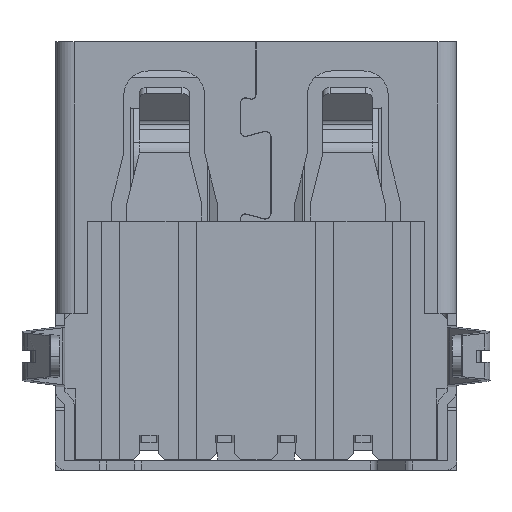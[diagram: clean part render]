
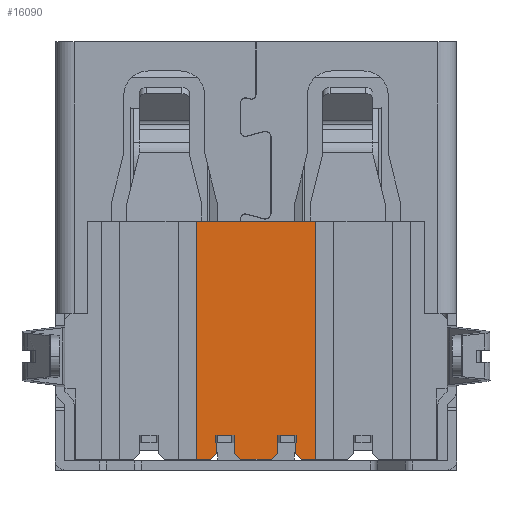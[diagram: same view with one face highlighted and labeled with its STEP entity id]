
A CAD part, front view. The second image highlights one B-rep face of the part: STEP entity #16090.
In plain terms, the highlighted planar face has unit normal (0, -1, 0).
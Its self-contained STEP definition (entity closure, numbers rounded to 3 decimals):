
#29 = DIRECTION ( 'NONE',  ( 1., 0., 0. ) ) ;
#78 = LINE ( 'NONE', #5264, #2960 ) ;
#275 = EDGE_CURVE ( 'NONE', #8951, #6910, #13512, .T. ) ;
#581 = CARTESIAN_POINT ( 'NONE',  ( 3.98, -6.1, 6.95 ) ) ;
#896 = CARTESIAN_POINT ( 'NONE',  ( -3.02, -6.1, 4.3 ) ) ;
#1021 = VERTEX_POINT ( 'NONE', #1642 ) ;
#1056 = VERTEX_POINT ( 'NONE', #20363 ) ;
#1101 = VECTOR ( 'NONE', #15560, 1000. ) ;
#1265 = LINE ( 'NONE', #12052, #1101 ) ;
#1316 = CARTESIAN_POINT ( 'NONE',  ( 4.77, -6.1, 7.75 ) ) ;
#1438 = CARTESIAN_POINT ( 'NONE',  ( 3.98, -6.1, 0. ) ) ;
#1642 = CARTESIAN_POINT ( 'NONE',  ( 4.57, -6.1, 5.55 ) ) ;
#1750 = CARTESIAN_POINT ( 'NONE',  ( 4.77, -6.1, 4.75 ) ) ;
#1772 = CARTESIAN_POINT ( 'NONE',  ( 4.77, -6.1, 4.75 ) ) ;
#1869 = DIRECTION ( 'NONE',  ( 0., 0., -1. ) ) ;
#2096 = ORIENTED_EDGE ( 'NONE', *, *, #8460, .T. ) ;
#2363 = ORIENTED_EDGE ( 'NONE', *, *, #4243, .T. ) ;
#2655 = DIRECTION ( 'NONE',  ( 0., 0., -1. ) ) ;
#2670 = VECTOR ( 'NONE', #2655, 1000. ) ;
#2960 = VECTOR ( 'NONE', #1869, 1000. ) ;
#3129 = VECTOR ( 'NONE', #16222, 1000. ) ;
#3176 = VECTOR ( 'NONE', #18240, 1000. ) ;
#3221 = CARTESIAN_POINT ( 'NONE',  ( 4.57, -6.1, 6.95 ) ) ;
#3343 = EDGE_CURVE ( 'NONE', #1056, #14543, #18358, .T. ) ;
#3367 = LINE ( 'NONE', #1438, #10193 ) ;
#3455 = DIRECTION ( 'NONE',  ( 0., 0., 1. ) ) ;
#3516 = VECTOR ( 'NONE', #7206, 1000. ) ;
#3611 = VERTEX_POINT ( 'NONE', #3221 ) ;
#3681 = LINE ( 'NONE', #1750, #3516 ) ;
#3686 = ORIENTED_EDGE ( 'NONE', *, *, #3343, .F. ) ;
#3790 = VERTEX_POINT ( 'NONE', #5276 ) ;
#3814 = PLANE ( 'NONE',  #8812 ) ;
#3917 = VECTOR ( 'NONE', #6950, 1000. ) ;
#4243 = EDGE_CURVE ( 'NONE', #14569, #1021, #9341, .T. ) ;
#4336 = VECTOR ( 'NONE', #13407, 1000. ) ;
#4423 = DIRECTION ( 'NONE',  ( 1., 0., 0. ) ) ;
#4478 = LINE ( 'NONE', #4593, #2670 ) ;
#4593 = CARTESIAN_POINT ( 'NONE',  ( 4.77, -6.1, 0. ) ) ;
#4780 = ORIENTED_EDGE ( 'NONE', *, *, #21063, .T. ) ;
#5206 = CARTESIAN_POINT ( 'NONE',  ( 4.77, -6.1, 6.75 ) ) ;
#5232 = VECTOR ( 'NONE', #4423, 1000. ) ;
#5264 = CARTESIAN_POINT ( 'NONE',  ( 4.77, -6.1, 0. ) ) ;
#5274 = DIRECTION ( 'NONE',  ( 0., -1., 0. ) ) ;
#5276 = CARTESIAN_POINT ( 'NONE',  ( -3.02, -6.1, 8.2 ) ) ;
#5293 = LINE ( 'NONE', #1316, #3176 ) ;
#5382 = EDGE_CURVE ( 'NONE', #16556, #3790, #16259, .T. ) ;
#5422 = ORIENTED_EDGE ( 'NONE', *, *, #5382, .F. ) ;
#6002 = CARTESIAN_POINT ( 'NONE',  ( 3.99, -6.1, 7.55 ) ) ;
#6043 = CARTESIAN_POINT ( 'NONE',  ( 4.77, -6.1, 4.3 ) ) ;
#6135 = LINE ( 'NONE', #8081, #4336 ) ;
#6234 = VERTEX_POINT ( 'NONE', #16055 ) ;
#6910 = VERTEX_POINT ( 'NONE', #22649 ) ;
#6950 = DIRECTION ( 'NONE',  ( 0., 0., 1. ) ) ;
#7073 = VECTOR ( 'NONE', #14812, 1000. ) ;
#7206 = DIRECTION ( 'NONE',  ( 0.707, 0., -0.707 ) ) ;
#7263 = CARTESIAN_POINT ( 'NONE',  ( 4.77, -6.1, 4.95 ) ) ;
#7608 = CARTESIAN_POINT ( 'NONE',  ( 4.77, -6.1, 0. ) ) ;
#7989 = EDGE_CURVE ( 'NONE', #1056, #3790, #16617, .T. ) ;
#8081 = CARTESIAN_POINT ( 'NONE',  ( 4.77, -6.1, 5.75 ) ) ;
#8447 = VECTOR ( 'NONE', #18593, 1000. ) ;
#8449 = ORIENTED_EDGE ( 'NONE', *, *, #23079, .F. ) ;
#8460 = EDGE_CURVE ( 'NONE', #6234, #14569, #3367, .T. ) ;
#8701 = DIRECTION ( 'NONE',  ( 0., 0., 1. ) ) ;
#8715 = ORIENTED_EDGE ( 'NONE', *, *, #16036, .F. ) ;
#8812 = AXIS2_PLACEMENT_3D ( 'NONE', #21839, #5274, #18097 ) ;
#8951 = VERTEX_POINT ( 'NONE', #14356 ) ;
#9038 = CARTESIAN_POINT ( 'NONE',  ( 4.77, -6.1, 6.75 ) ) ;
#9104 = ORIENTED_EDGE ( 'NONE', *, *, #275, .T. ) ;
#9330 = ORIENTED_EDGE ( 'NONE', *, *, #13813, .F. ) ;
#9341 = LINE ( 'NONE', #17062, #22764 ) ;
#9972 = ORIENTED_EDGE ( 'NONE', *, *, #7989, .T. ) ;
#10193 = VECTOR ( 'NONE', #8701, 1000. ) ;
#11140 = LINE ( 'NONE', #7263, #16225 ) ;
#11754 = FACE_OUTER_BOUND ( 'NONE', #20525, .T. ) ;
#12035 = ORIENTED_EDGE ( 'NONE', *, *, #23429, .F. ) ;
#12052 = CARTESIAN_POINT ( 'NONE',  ( 4.77, -6.1, 6.95 ) ) ;
#12196 = CARTESIAN_POINT ( 'NONE',  ( 3.98, -6.1, 0. ) ) ;
#13407 = DIRECTION ( 'NONE',  ( -0.707, 0., -0.707 ) ) ;
#13489 = VERTEX_POINT ( 'NONE', #581 ) ;
#13512 = LINE ( 'NONE', #6002, #5232 ) ;
#13813 = EDGE_CURVE ( 'NONE', #17112, #14285, #78, .T. ) ;
#13965 = ORIENTED_EDGE ( 'NONE', *, *, #23512, .T. ) ;
#14285 = VERTEX_POINT ( 'NONE', #6043 ) ;
#14356 = CARTESIAN_POINT ( 'NONE',  ( 3.98, -6.1, 7.55 ) ) ;
#14543 = VERTEX_POINT ( 'NONE', #16319 ) ;
#14569 = VERTEX_POINT ( 'NONE', #23914 ) ;
#14772 = VERTEX_POINT ( 'NONE', #21362 ) ;
#14812 = DIRECTION ( 'NONE',  ( -1., 0., 0. ) ) ;
#14923 = ORIENTED_EDGE ( 'NONE', *, *, #22459, .F. ) ;
#14987 = VERTEX_POINT ( 'NONE', #9038 ) ;
#15304 = EDGE_CURVE ( 'NONE', #3611, #13489, #1265, .T. ) ;
#15331 = ORIENTED_EDGE ( 'NONE', *, *, #18190, .F. ) ;
#15560 = DIRECTION ( 'NONE',  ( -1., 0., 0. ) ) ;
#16036 = EDGE_CURVE ( 'NONE', #14987, #18044, #4478, .T. ) ;
#16055 = CARTESIAN_POINT ( 'NONE',  ( 3.98, -6.1, 4.95 ) ) ;
#16090 = ADVANCED_FACE ( 'NONE', ( #11754 ), #3814, .T. ) ;
#16222 = DIRECTION ( 'NONE',  ( 0.707, 0., -0.707 ) ) ;
#16225 = VECTOR ( 'NONE', #18491, 1000. ) ;
#16259 = LINE ( 'NONE', #21569, #3917 ) ;
#16319 = CARTESIAN_POINT ( 'NONE',  ( 4.77, -6.1, 7.75 ) ) ;
#16556 = VERTEX_POINT ( 'NONE', #896 ) ;
#16617 = LINE ( 'NONE', #22289, #7073 ) ;
#17062 = CARTESIAN_POINT ( 'NONE',  ( 3.99, -6.1, 5.55 ) ) ;
#17112 = VERTEX_POINT ( 'NONE', #1772 ) ;
#17275 = ORIENTED_EDGE ( 'NONE', *, *, #20533, .T. ) ;
#17458 = LINE ( 'NONE', #21202, #22625 ) ;
#17540 = CARTESIAN_POINT ( 'NONE',  ( 4.77, -6.1, 5.75 ) ) ;
#18044 = VERTEX_POINT ( 'NONE', #17540 ) ;
#18097 = DIRECTION ( 'NONE',  ( 0., 0., -1. ) ) ;
#18190 = EDGE_CURVE ( 'NONE', #3611, #14987, #23339, .T. ) ;
#18240 = DIRECTION ( 'NONE',  ( -0.707, 0., -0.707 ) ) ;
#18358 = LINE ( 'NONE', #7608, #8447 ) ;
#18491 = DIRECTION ( 'NONE',  ( -1., 0., 0. ) ) ;
#18593 = DIRECTION ( 'NONE',  ( 0., 0., -1. ) ) ;
#20024 = LINE ( 'NONE', #12196, #23644 ) ;
#20039 = ORIENTED_EDGE ( 'NONE', *, *, #15304, .T. ) ;
#20363 = CARTESIAN_POINT ( 'NONE',  ( 4.77, -6.1, 8.2 ) ) ;
#20525 = EDGE_LOOP ( 'NONE', ( #12035, #8715, #15331, #20039, #13965, #9104, #8449, #3686, #9972, #5422, #4780, #9330, #14923, #17275, #2096, #2363 ) ) ;
#20533 = EDGE_CURVE ( 'NONE', #14772, #6234, #11140, .T. ) ;
#21063 = EDGE_CURVE ( 'NONE', #16556, #14285, #17458, .T. ) ;
#21202 = CARTESIAN_POINT ( 'NONE',  ( 0., -6.1, 4.3 ) ) ;
#21362 = CARTESIAN_POINT ( 'NONE',  ( 4.57, -6.1, 4.95 ) ) ;
#21569 = CARTESIAN_POINT ( 'NONE',  ( -3.02, -6.1, 0. ) ) ;
#21839 = CARTESIAN_POINT ( 'NONE',  ( 0., -6.1, 0. ) ) ;
#22289 = CARTESIAN_POINT ( 'NONE',  ( 0., -6.1, 8.2 ) ) ;
#22459 = EDGE_CURVE ( 'NONE', #14772, #17112, #3681, .T. ) ;
#22625 = VECTOR ( 'NONE', #23012, 1000. ) ;
#22649 = CARTESIAN_POINT ( 'NONE',  ( 4.57, -6.1, 7.55 ) ) ;
#22764 = VECTOR ( 'NONE', #29, 1000. ) ;
#23012 = DIRECTION ( 'NONE',  ( 1., 0., 0. ) ) ;
#23079 = EDGE_CURVE ( 'NONE', #14543, #6910, #5293, .T. ) ;
#23339 = LINE ( 'NONE', #5206, #3129 ) ;
#23429 = EDGE_CURVE ( 'NONE', #18044, #1021, #6135, .T. ) ;
#23512 = EDGE_CURVE ( 'NONE', #13489, #8951, #20024, .T. ) ;
#23644 = VECTOR ( 'NONE', #3455, 1000. ) ;
#23914 = CARTESIAN_POINT ( 'NONE',  ( 3.98, -6.1, 5.55 ) ) ;
